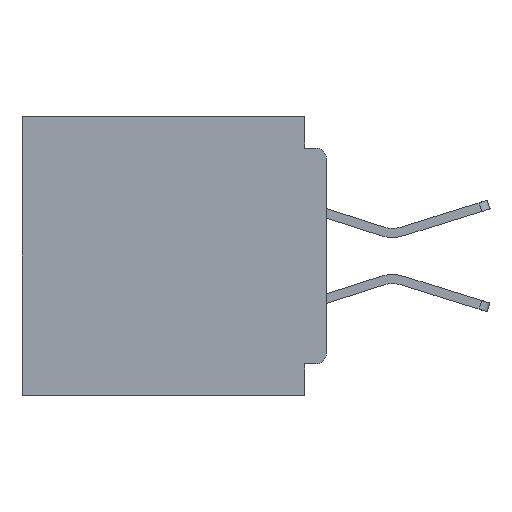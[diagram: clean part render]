
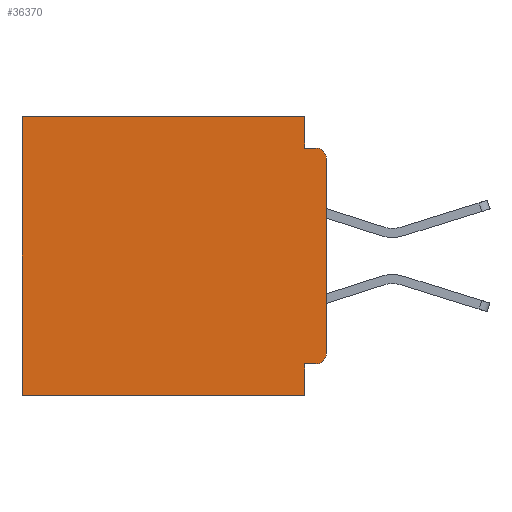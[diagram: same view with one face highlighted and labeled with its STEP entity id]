
A CAD part, left-side view. The second image highlights one B-rep face of the part: STEP entity #36370.
In plain terms, the highlighted planar face has unit normal (-1, 0, 0).
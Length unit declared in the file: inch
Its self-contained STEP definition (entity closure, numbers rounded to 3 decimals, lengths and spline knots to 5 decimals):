
#69 = CARTESIAN_POINT ( 'NONE',  ( 0.3, 0.031, 0. ) ) ;
#230 = CARTESIAN_POINT ( 'NONE',  ( 0.3, 0., -0.4 ) ) ;
#790 = ORIENTED_EDGE ( 'NONE', *, *, #27288, .T. ) ;
#835 = EDGE_CURVE ( 'NONE', #24213, #6905, #4114, .T. ) ;
#1864 = ORIENTED_EDGE ( 'NONE', *, *, #37782, .F. ) ;
#2597 = VERTEX_POINT ( 'NONE', #37072 ) ;
#3669 = DIRECTION ( 'NONE',  ( 0., 0., -1. ) ) ;
#4114 = LINE ( 'NONE', #38625, #39962 ) ;
#5208 = EDGE_CURVE ( 'NONE', #16285, #6905, #17255, .T. ) ;
#5685 = VECTOR ( 'NONE', #15481, 39.37008 ) ;
#6047 = LINE ( 'NONE', #39051, #24005 ) ;
#6125 = VERTEX_POINT ( 'NONE', #20071 ) ;
#6482 = DIRECTION ( 'NONE',  ( 0., 0., -1. ) ) ;
#6905 = VERTEX_POINT ( 'NONE', #42506 ) ;
#6986 = FACE_OUTER_BOUND ( 'NONE', #31720, .T. ) ;
#7036 = EDGE_CURVE ( 'NONE', #22147, #12905, #35563, .T. ) ;
#8801 = CARTESIAN_POINT ( 'NONE',  ( 0.3, 0.015, -0.34 ) ) ;
#9804 = CARTESIAN_POINT ( 'NONE',  ( 0.3, 0.015, -0.06 ) ) ;
#10317 = CARTESIAN_POINT ( 'NONE',  ( 0.3, 0., -0.045 ) ) ;
#10322 = ORIENTED_EDGE ( 'NONE', *, *, #26898, .F. ) ;
#10422 = DIRECTION ( 'NONE',  ( 0., 0., -1. ) ) ;
#11884 = CARTESIAN_POINT ( 'NONE',  ( 0.3, 0., 0. ) ) ;
#12387 = DIRECTION ( 'NONE',  ( 0., 0., -1. ) ) ;
#12440 = VERTEX_POINT ( 'NONE', #13678 ) ;
#12905 = VERTEX_POINT ( 'NONE', #19713 ) ;
#12987 = VECTOR ( 'NONE', #6482, 39.37008 ) ;
#13421 = DIRECTION ( 'NONE',  ( 0., 0., -1. ) ) ;
#13678 = CARTESIAN_POINT ( 'NONE',  ( 0.3, 0.015, -0.355 ) ) ;
#13754 = AXIS2_PLACEMENT_3D ( 'NONE', #8801, #33855, #12387 ) ;
#14150 = CARTESIAN_POINT ( 'NONE',  ( 0.3, 0., -0.34 ) ) ;
#15481 = DIRECTION ( 'NONE',  ( 0., 1., 0. ) ) ;
#15717 = LINE ( 'NONE', #10317, #43132 ) ;
#16285 = VERTEX_POINT ( 'NONE', #39252 ) ;
#17255 = LINE ( 'NONE', #41816, #45735 ) ;
#17311 = AXIS2_PLACEMENT_3D ( 'NONE', #230, #43298, #21901 ) ;
#19713 = CARTESIAN_POINT ( 'NONE',  ( 0.3, 0.031, -0.045 ) ) ;
#20071 = CARTESIAN_POINT ( 'NONE',  ( 0.3, 0.031, -0.355 ) ) ;
#21292 = CARTESIAN_POINT ( 'NONE',  ( 0.3, 0.031, -0.4 ) ) ;
#21436 = CARTESIAN_POINT ( 'NONE',  ( 0.3, 0., -0.355 ) ) ;
#21901 = DIRECTION ( 'NONE',  ( 0., 0., -1. ) ) ;
#22147 = VERTEX_POINT ( 'NONE', #29121 ) ;
#22513 = LINE ( 'NONE', #35122, #12987 ) ;
#22709 = VECTOR ( 'NONE', #3669, 39.37008 ) ;
#23741 = ORIENTED_EDGE ( 'NONE', *, *, #43640, .T. ) ;
#24005 = VECTOR ( 'NONE', #10422, 39.37008 ) ;
#24213 = VERTEX_POINT ( 'NONE', #21292 ) ;
#24764 = LINE ( 'NONE', #11884, #5685 ) ;
#24891 = CARTESIAN_POINT ( 'NONE',  ( 0.3, 0., -0.06 ) ) ;
#25984 = AXIS2_PLACEMENT_3D ( 'NONE', #9804, #34843, #13421 ) ;
#26898 = EDGE_CURVE ( 'NONE', #6125, #24213, #22513, .T. ) ;
#27013 = VERTEX_POINT ( 'NONE', #14150 ) ;
#27288 = EDGE_CURVE ( 'NONE', #12440, #27013, #35343, .T. ) ;
#27561 = EDGE_CURVE ( 'NONE', #12905, #2597, #15717, .T. ) ;
#27608 = VERTEX_POINT ( 'NONE', #24891 ) ;
#28671 = LINE ( 'NONE', #21436, #45426 ) ;
#29121 = CARTESIAN_POINT ( 'NONE',  ( 0.3, 0.031, 0. ) ) ;
#29285 = ORIENTED_EDGE ( 'NONE', *, *, #27561, .F. ) ;
#29907 = ORIENTED_EDGE ( 'NONE', *, *, #835, .F. ) ;
#31720 = EDGE_LOOP ( 'NONE', ( #45450, #36531, #29285, #39365, #23741, #42725, #29907, #10322, #1864, #790 ) ) ;
#32072 = DIRECTION ( 'NONE',  ( 0., 1., 0. ) ) ;
#33855 = DIRECTION ( 'NONE',  ( -1., 0., 0. ) ) ;
#34843 = DIRECTION ( 'NONE',  ( -1., 0., 0. ) ) ;
#35122 = CARTESIAN_POINT ( 'NONE',  ( 0.3, 0.031, -0.4 ) ) ;
#35230 = DIRECTION ( 'NONE',  ( 0., -1., 0. ) ) ;
#35343 = CIRCLE ( 'NONE', #13754, 0.015 ) ;
#35563 = LINE ( 'NONE', #69, #22709 ) ;
#36370 = ADVANCED_FACE ( 'NONE', ( #6986 ), #39696, .F. ) ;
#36531 = ORIENTED_EDGE ( 'NONE', *, *, #36761, .T. ) ;
#36761 = EDGE_CURVE ( 'NONE', #27608, #2597, #43862, .T. ) ;
#37072 = CARTESIAN_POINT ( 'NONE',  ( 0.3, 0.015, -0.045 ) ) ;
#37782 = EDGE_CURVE ( 'NONE', #12440, #6125, #28671, .T. ) ;
#38625 = CARTESIAN_POINT ( 'NONE',  ( 0.3, 0., -0.4 ) ) ;
#39025 = DIRECTION ( 'NONE',  ( 0., 1., 0. ) ) ;
#39051 = CARTESIAN_POINT ( 'NONE',  ( 0.3, 0., -0.4 ) ) ;
#39252 = CARTESIAN_POINT ( 'NONE',  ( 0.3, 0.437, 0. ) ) ;
#39365 = ORIENTED_EDGE ( 'NONE', *, *, #7036, .F. ) ;
#39696 = PLANE ( 'NONE',  #17311 ) ;
#39962 = VECTOR ( 'NONE', #39025, 39.37008 ) ;
#40717 = EDGE_CURVE ( 'NONE', #27608, #27013, #6047, .T. ) ;
#41816 = CARTESIAN_POINT ( 'NONE',  ( 0.3, 0.437, -0.4 ) ) ;
#42062 = DIRECTION ( 'NONE',  ( 0., 0., -1. ) ) ;
#42506 = CARTESIAN_POINT ( 'NONE',  ( 0.3, 0.437, -0.4 ) ) ;
#42725 = ORIENTED_EDGE ( 'NONE', *, *, #5208, .T. ) ;
#43132 = VECTOR ( 'NONE', #35230, 39.37008 ) ;
#43298 = DIRECTION ( 'NONE',  ( 1., 0., 0. ) ) ;
#43640 = EDGE_CURVE ( 'NONE', #22147, #16285, #24764, .T. ) ;
#43862 = CIRCLE ( 'NONE', #25984, 0.015 ) ;
#45426 = VECTOR ( 'NONE', #32072, 39.37008 ) ;
#45450 = ORIENTED_EDGE ( 'NONE', *, *, #40717, .F. ) ;
#45735 = VECTOR ( 'NONE', #42062, 39.37008 ) ;
